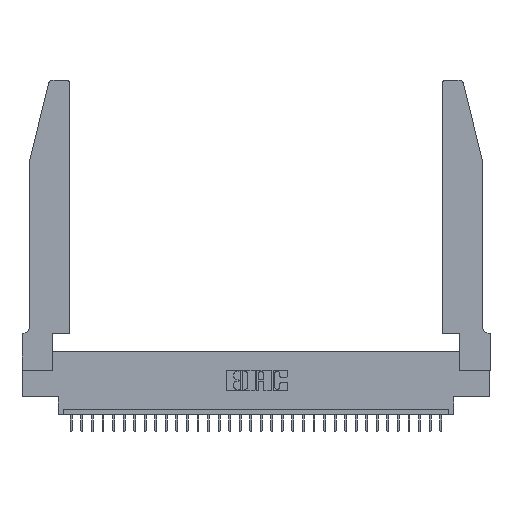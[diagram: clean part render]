
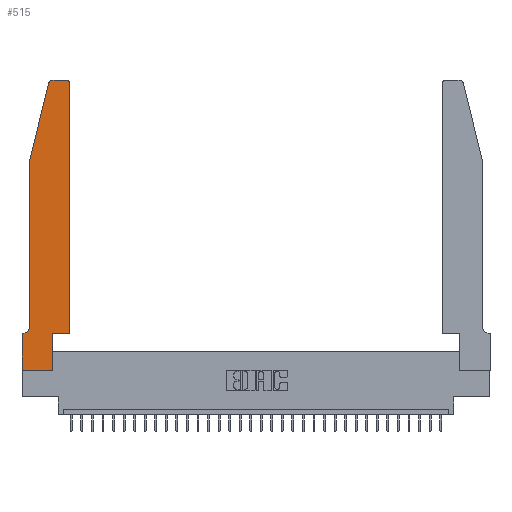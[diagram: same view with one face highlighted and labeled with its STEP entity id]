
A CAD part, top view. The second image highlights one B-rep face of the part: STEP entity #515.
In plain terms, the highlighted planar face has unit normal (0, 0, 1).
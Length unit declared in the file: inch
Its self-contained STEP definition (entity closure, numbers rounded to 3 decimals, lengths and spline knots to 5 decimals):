
#108 = CARTESIAN_POINT ( 'NONE',  ( 0.4505, 2.72, 0.37 ) ) ;
#130 = EDGE_CURVE ( 'NONE', #8840, #10737, #30368, .T. ) ;
#212 = EDGE_CURVE ( 'NONE', #11888, #29707, #9403, .T. ) ;
#272 = DIRECTION ( 'NONE',  ( 0., 1., 0. ) ) ;
#515 = ADVANCED_FACE ( 'NONE', ( #2214 ), #17233, .T. ) ;
#1340 = ORIENTED_EDGE ( 'NONE', *, *, #20670, .T. ) ;
#1349 = DIRECTION ( 'NONE',  ( -0.239, -0.971, 0. ) ) ;
#1364 = VECTOR ( 'NONE', #7262, 39.37008 ) ;
#1425 = ORIENTED_EDGE ( 'NONE', *, *, #4559, .T. ) ;
#1708 = LINE ( 'NONE', #2222, #14057 ) ;
#1808 = CARTESIAN_POINT ( 'NONE',  ( 0.2865, 0.35, 0.37 ) ) ;
#2023 = EDGE_CURVE ( 'NONE', #13707, #11513, #1708, .T. ) ;
#2125 = CARTESIAN_POINT ( 'NONE',  ( 0.0055, 0.35, 0.37 ) ) ;
#2214 = FACE_OUTER_BOUND ( 'NONE', #12369, .T. ) ;
#2222 = CARTESIAN_POINT ( 'NONE',  ( 0., 0., 0.37 ) ) ;
#2872 = CARTESIAN_POINT ( 'NONE',  ( 0.4205, 2.72, 0.37 ) ) ;
#2898 = EDGE_CURVE ( 'NONE', #11513, #29957, #3259, .T. ) ;
#3004 = VECTOR ( 'NONE', #25585, 39.37008 ) ;
#3259 = LINE ( 'NONE', #20280, #30553 ) ;
#3518 = CARTESIAN_POINT ( 'NONE',  ( 0.284, 2.72, 0.37 ) ) ;
#3794 = CARTESIAN_POINT ( 'NONE',  ( 0., 0., 0.37 ) ) ;
#4157 = DIRECTION ( 'NONE',  ( -1., 0., 0. ) ) ;
#4180 = VECTOR ( 'NONE', #272, 39.37008 ) ;
#4559 = EDGE_CURVE ( 'NONE', #10629, #21135, #31681, .T. ) ;
#4569 = DIRECTION ( 'NONE',  ( 1., 0., 0. ) ) ;
#4585 = CARTESIAN_POINT ( 'NONE',  ( 0.0755, 2., 0.37 ) ) ;
#5440 = DIRECTION ( 'NONE',  ( 1., 0., 0. ) ) ;
#6073 = DIRECTION ( 'NONE',  ( 1., 0., 0. ) ) ;
#6165 = LINE ( 'NONE', #25465, #4180 ) ;
#6335 = EDGE_CURVE ( 'NONE', #10737, #11888, #15518, .T. ) ;
#7262 = DIRECTION ( 'NONE',  ( 0., 1., 0. ) ) ;
#7924 = VECTOR ( 'NONE', #32243, 39.37008 ) ;
#8737 = CARTESIAN_POINT ( 'NONE',  ( 0.0755, 2., 0.37 ) ) ;
#8840 = VERTEX_POINT ( 'NONE', #24832 ) ;
#9012 = LINE ( 'NONE', #17002, #16575 ) ;
#9129 = CARTESIAN_POINT ( 'NONE',  ( 0.284, 2.75, 0.37 ) ) ;
#9403 = CIRCLE ( 'NONE', #12719, 0.07 ) ;
#9480 = CARTESIAN_POINT ( 'NONE',  ( 0.0055, 0.42, 0.37 ) ) ;
#9780 = LINE ( 'NONE', #15118, #1364 ) ;
#10181 = ORIENTED_EDGE ( 'NONE', *, *, #2023, .T. ) ;
#10542 = DIRECTION ( 'NONE',  ( 0., -1., 0. ) ) ;
#10629 = VERTEX_POINT ( 'NONE', #27321 ) ;
#10724 = VERTEX_POINT ( 'NONE', #1808 ) ;
#10737 = VERTEX_POINT ( 'NONE', #30044 ) ;
#11390 = VECTOR ( 'NONE', #1349, 39.37008 ) ;
#11513 = VERTEX_POINT ( 'NONE', #3794 ) ;
#11888 = VERTEX_POINT ( 'NONE', #13928 ) ;
#12279 = ORIENTED_EDGE ( 'NONE', *, *, #2898, .T. ) ;
#12331 = CARTESIAN_POINT ( 'NONE',  ( 0.2605, 2.75, 0.37 ) ) ;
#12369 = EDGE_LOOP ( 'NONE', ( #1425, #19549, #26025, #27969, #32057, #25892, #10181, #12279, #30683, #1340, #12833, #15550 ) ) ;
#12719 = AXIS2_PLACEMENT_3D ( 'NONE', #9480, #17042, #4157 ) ;
#12833 = ORIENTED_EDGE ( 'NONE', *, *, #15560, .T. ) ;
#13368 = CARTESIAN_POINT ( 'NONE',  ( 0.4505, 0.35, 0.37 ) ) ;
#13575 = CARTESIAN_POINT ( 'NONE',  ( 0.2865, 0., 0.37 ) ) ;
#13707 = VERTEX_POINT ( 'NONE', #15579 ) ;
#13928 = CARTESIAN_POINT ( 'NONE',  ( 0.0755, 0.42, 0.37 ) ) ;
#14048 = DIRECTION ( 'NONE',  ( 0., 0., 1. ) ) ;
#14057 = VECTOR ( 'NONE', #19987, 39.37008 ) ;
#14333 = VECTOR ( 'NONE', #10542, 39.37008 ) ;
#15116 = EDGE_CURVE ( 'NONE', #29707, #13707, #20474, .T. ) ;
#15118 = CARTESIAN_POINT ( 'NONE',  ( 0.4505, 0.35, 0.37 ) ) ;
#15518 = LINE ( 'NONE', #4585, #14333 ) ;
#15550 = ORIENTED_EDGE ( 'NONE', *, *, #27103, .T. ) ;
#15560 = EDGE_CURVE ( 'NONE', #28269, #25660, #9780, .T. ) ;
#15579 = CARTESIAN_POINT ( 'NONE',  ( 0., 0.35, 0.37 ) ) ;
#15990 = DIRECTION ( 'NONE',  ( 1., 0., 0. ) ) ;
#16114 = EDGE_CURVE ( 'NONE', #29957, #10724, #6165, .T. ) ;
#16575 = VECTOR ( 'NONE', #27118, 39.37008 ) ;
#17002 = CARTESIAN_POINT ( 'NONE',  ( 0.4505, 0.35, 0.37 ) ) ;
#17042 = DIRECTION ( 'NONE',  ( 0., 0., -1. ) ) ;
#17233 = PLANE ( 'NONE',  #23139 ) ;
#19549 = ORIENTED_EDGE ( 'NONE', *, *, #24120, .T. ) ;
#19768 = CARTESIAN_POINT ( 'NONE',  ( 0., 0.35, 0.37 ) ) ;
#19987 = DIRECTION ( 'NONE',  ( 0., -1., 0. ) ) ;
#20075 = AXIS2_PLACEMENT_3D ( 'NONE', #2872, #20612, #5440 ) ;
#20280 = CARTESIAN_POINT ( 'NONE',  ( 0., 0., 0.37 ) ) ;
#20474 = LINE ( 'NONE', #25814, #3004 ) ;
#20612 = DIRECTION ( 'NONE',  ( 0., 0., 1. ) ) ;
#20670 = EDGE_CURVE ( 'NONE', #10724, #28269, #9012, .T. ) ;
#20885 = AXIS2_PLACEMENT_3D ( 'NONE', #3518, #14048, #6073 ) ;
#21135 = VERTEX_POINT ( 'NONE', #9129 ) ;
#21216 = CIRCLE ( 'NONE', #20075, 0.03 ) ;
#23139 = AXIS2_PLACEMENT_3D ( 'NONE', #19768, #24716, #4569 ) ;
#24120 = EDGE_CURVE ( 'NONE', #21135, #8840, #31725, .T. ) ;
#24716 = DIRECTION ( 'NONE',  ( 0., 0., 1. ) ) ;
#24832 = CARTESIAN_POINT ( 'NONE',  ( 0.25487, 2.72718, 0.37 ) ) ;
#25465 = CARTESIAN_POINT ( 'NONE',  ( 0.2865, 0.35, 0.37 ) ) ;
#25585 = DIRECTION ( 'NONE',  ( -1., 0., 0. ) ) ;
#25660 = VERTEX_POINT ( 'NONE', #108 ) ;
#25814 = CARTESIAN_POINT ( 'NONE',  ( 0.0755, 0.35, 0.37 ) ) ;
#25892 = ORIENTED_EDGE ( 'NONE', *, *, #15116, .T. ) ;
#26025 = ORIENTED_EDGE ( 'NONE', *, *, #130, .T. ) ;
#27103 = EDGE_CURVE ( 'NONE', #25660, #10629, #21216, .T. ) ;
#27118 = DIRECTION ( 'NONE',  ( 1., 0., 0. ) ) ;
#27321 = CARTESIAN_POINT ( 'NONE',  ( 0.4205, 2.75, 0.37 ) ) ;
#27969 = ORIENTED_EDGE ( 'NONE', *, *, #6335, .T. ) ;
#28269 = VERTEX_POINT ( 'NONE', #13368 ) ;
#29707 = VERTEX_POINT ( 'NONE', #2125 ) ;
#29957 = VERTEX_POINT ( 'NONE', #13575 ) ;
#30044 = CARTESIAN_POINT ( 'NONE',  ( 0.0755, 2., 0.37 ) ) ;
#30368 = LINE ( 'NONE', #8737, #11390 ) ;
#30553 = VECTOR ( 'NONE', #15990, 39.37008 ) ;
#30683 = ORIENTED_EDGE ( 'NONE', *, *, #16114, .T. ) ;
#31681 = LINE ( 'NONE', #12331, #7924 ) ;
#31725 = CIRCLE ( 'NONE', #20885, 0.03 ) ;
#32057 = ORIENTED_EDGE ( 'NONE', *, *, #212, .T. ) ;
#32243 = DIRECTION ( 'NONE',  ( -1., 0., 0. ) ) ;
